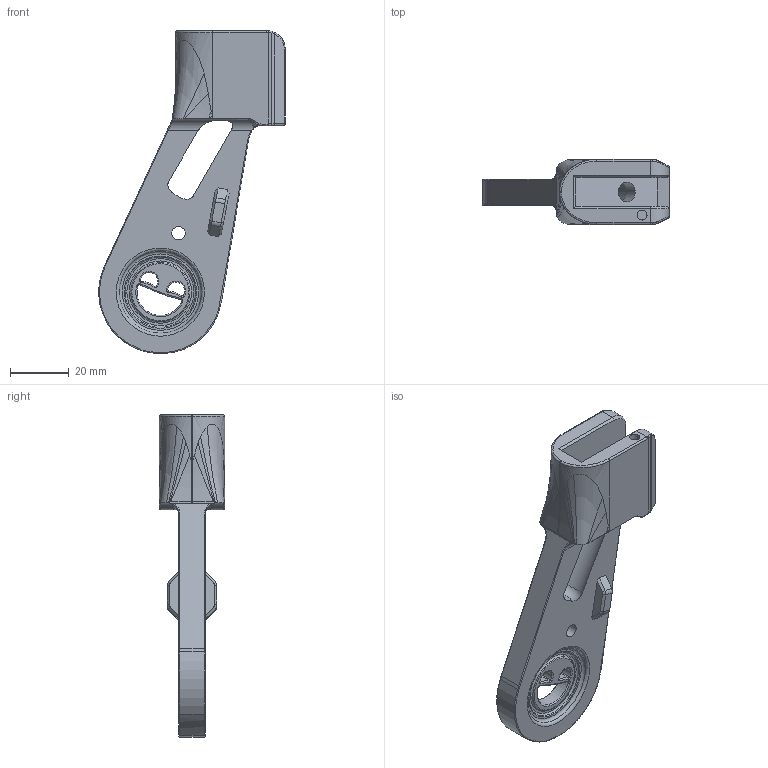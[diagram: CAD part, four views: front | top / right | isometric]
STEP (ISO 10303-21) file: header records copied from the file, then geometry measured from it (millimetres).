
FILE_DESCRIPTION(/* description */ (''),/* implementation_level */ '2;1');
FILE_NAME(/* name */ 'Grip Frame.step',/* time_stamp */ '2021-09-21T09:18:18-04:00',/* author */ (''),/* organization */ (''),/* preprocessor_version */ 'ST-DEVELOPER v18.1',/* originating_system */ 'Autodesk Translation Framework v10.10.0.1391',/* authorisation */ '');
FILE_SCHEMA (('AUTOMOTIVE_DESIGN { 1 0 10303 214 3 1 1 }'));
Length unit declared in the file: millimetre
Products named in the file (1): Grip Frame
Bounding box: 63.47 x 22.23 x 109.88 mm (x, y, z)
Volume: 35882.7 mm3; surface area: 14142.7 mm2
Topology: 1 solids, 1 shells, 235 faces, 573 edges, 345 vertices
Faces by surface type: bspline 82, plane 55, cylinder 51, torus 36, cone 11
Full cylindrical faces by diameter (mm): 3.4 x1, 4.6 x1, 6.8 x1, 13.165 x1
Entity records: 10260 total; most frequent: CARTESIAN_POINT 5180, ORIENTED_EDGE 1142, DIRECTION 896, EDGE_CURVE 571, AXIS2_PLACEMENT_3D 361, VERTEX_POINT 345, EDGE_LOOP 254, FACE_OUTER_BOUND 235
